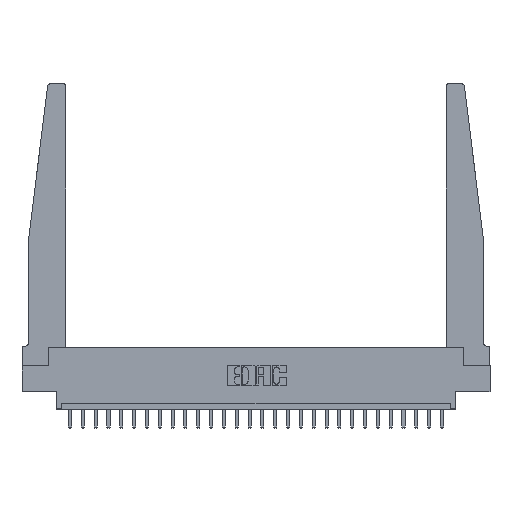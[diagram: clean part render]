
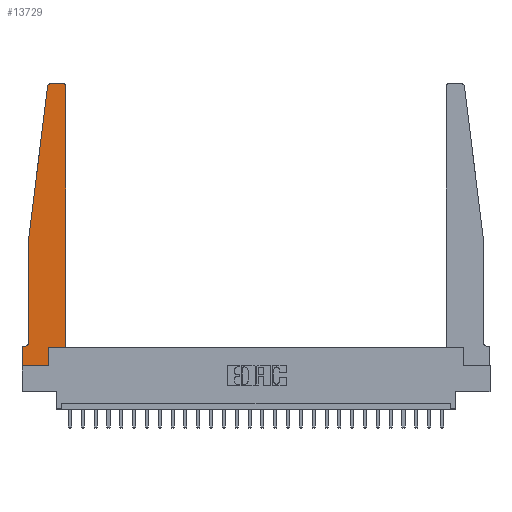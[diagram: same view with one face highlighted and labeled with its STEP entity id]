
A CAD part, top view. The second image highlights one B-rep face of the part: STEP entity #13729.
In plain terms, the highlighted planar face has unit normal (0, 0, 1).
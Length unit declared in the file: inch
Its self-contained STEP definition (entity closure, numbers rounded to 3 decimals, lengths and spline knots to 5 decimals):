
#373 = ORIENTED_EDGE ( 'NONE', *, *, #19788, .T. ) ;
#397 = CARTESIAN_POINT ( 'NONE',  ( 0.27653, 2.72, 0.37 ) ) ;
#616 = AXIS2_PLACEMENT_3D ( 'NONE', #15666, #13822, #25387 ) ;
#745 = LINE ( 'NONE', #6727, #14273 ) ;
#876 = VERTEX_POINT ( 'NONE', #17961 ) ;
#1001 = DIRECTION ( 'NONE',  ( 0., -1., 0. ) ) ;
#1969 = EDGE_CURVE ( 'NONE', #15614, #10396, #3071, .T. ) ;
#2006 = CARTESIAN_POINT ( 'NONE',  ( 0.065, 0.2375, 0.37 ) ) ;
#2117 = LINE ( 'NONE', #25653, #13832 ) ;
#2193 = VERTEX_POINT ( 'NONE', #17862 ) ;
#2628 = AXIS2_PLACEMENT_3D ( 'NONE', #17552, #11711, #25481 ) ;
#2677 = EDGE_CURVE ( 'NONE', #2193, #18642, #17796, .T. ) ;
#3039 = VECTOR ( 'NONE', #8495, 39.37008 ) ;
#3071 = LINE ( 'NONE', #18653, #11666 ) ;
#3136 = VECTOR ( 'NONE', #12286, 39.37008 ) ;
#3197 = ORIENTED_EDGE ( 'NONE', *, *, #13480, .T. ) ;
#3854 = VERTEX_POINT ( 'NONE', #13686 ) ;
#3909 = CARTESIAN_POINT ( 'NONE',  ( 0.425, 0.18, 0.37 ) ) ;
#4334 = ORIENTED_EDGE ( 'NONE', *, *, #24611, .T. ) ;
#4582 = FACE_OUTER_BOUND ( 'NONE', #11427, .T. ) ;
#4681 = ORIENTED_EDGE ( 'NONE', *, *, #14001, .T. ) ;
#4750 = CIRCLE ( 'NONE', #616, 0.03 ) ;
#5121 = ORIENTED_EDGE ( 'NONE', *, *, #21421, .T. ) ;
#6515 = DIRECTION ( 'NONE',  ( 0., 0., 1. ) ) ;
#6606 = CARTESIAN_POINT ( 'NONE',  ( 0.2605, 0.18, 0.37 ) ) ;
#6727 = CARTESIAN_POINT ( 'NONE',  ( 0.425, 0.18, 0.37 ) ) ;
#6967 = CARTESIAN_POINT ( 'NONE',  ( 0.2605, 0.18, 0.37 ) ) ;
#7396 = LINE ( 'NONE', #15320, #24579 ) ;
#7445 = CARTESIAN_POINT ( 'NONE',  ( 0.395, 2.75, 0.37 ) ) ;
#7620 = CIRCLE ( 'NONE', #2628, 0.05 ) ;
#8340 = CARTESIAN_POINT ( 'NONE',  ( 0.015, 0.1875, 0.37 ) ) ;
#8495 = DIRECTION ( 'NONE',  ( 1., 0., 0. ) ) ;
#8884 = ORIENTED_EDGE ( 'NONE', *, *, #10788, .T. ) ;
#9213 = DIRECTION ( 'NONE',  ( 0., 0., 1. ) ) ;
#10092 = CARTESIAN_POINT ( 'NONE',  ( 0.425, 2.72, 0.37 ) ) ;
#10161 = EDGE_CURVE ( 'NONE', #19123, #22030, #7620, .T. ) ;
#10373 = DIRECTION ( 'NONE',  ( 0., 1., 0. ) ) ;
#10396 = VERTEX_POINT ( 'NONE', #3909 ) ;
#10788 = EDGE_CURVE ( 'NONE', #10396, #21127, #745, .T. ) ;
#10823 = CARTESIAN_POINT ( 'NONE',  ( 0.2605, 0., 0.37 ) ) ;
#10944 = CARTESIAN_POINT ( 'NONE',  ( 0., 0., 0.37 ) ) ;
#11157 = AXIS2_PLACEMENT_3D ( 'NONE', #397, #6515, #16243 ) ;
#11427 = EDGE_LOOP ( 'NONE', ( #23142, #13453, #373, #4334, #13559, #3197, #15904, #20537, #4681, #17991, #8884, #5121 ) ) ;
#11666 = VECTOR ( 'NONE', #16470, 39.37008 ) ;
#11711 = DIRECTION ( 'NONE',  ( 0., 0., -1. ) ) ;
#12286 = DIRECTION ( 'NONE',  ( -1., 0., 0. ) ) ;
#13453 = ORIENTED_EDGE ( 'NONE', *, *, #2677, .T. ) ;
#13480 = EDGE_CURVE ( 'NONE', #22030, #14631, #14989, .T. ) ;
#13559 = ORIENTED_EDGE ( 'NONE', *, *, #10161, .T. ) ;
#13686 = CARTESIAN_POINT ( 'NONE',  ( 0., 0., 0.37 ) ) ;
#13729 = ADVANCED_FACE ( 'NONE', ( #4582 ), #22475, .T. ) ;
#13822 = DIRECTION ( 'NONE',  ( 0., 0., 1. ) ) ;
#13832 = VECTOR ( 'NONE', #14084, 39.37008 ) ;
#14001 = EDGE_CURVE ( 'NONE', #22856, #15614, #16473, .T. ) ;
#14084 = DIRECTION ( 'NONE',  ( 0., -1., 0. ) ) ;
#14273 = VECTOR ( 'NONE', #22545, 39.37008 ) ;
#14631 = VERTEX_POINT ( 'NONE', #19500 ) ;
#14854 = LINE ( 'NONE', #10944, #3039 ) ;
#14989 = LINE ( 'NONE', #20952, #18091 ) ;
#15122 = DIRECTION ( 'NONE',  ( -1., 0., 0. ) ) ;
#15217 = VECTOR ( 'NONE', #10373, 39.37008 ) ;
#15320 = CARTESIAN_POINT ( 'NONE',  ( 0.065, 1.25, 0.37 ) ) ;
#15614 = VERTEX_POINT ( 'NONE', #6967 ) ;
#15666 = CARTESIAN_POINT ( 'NONE',  ( 0.395, 2.72, 0.37 ) ) ;
#15904 = ORIENTED_EDGE ( 'NONE', *, *, #20406, .T. ) ;
#16202 = VERTEX_POINT ( 'NONE', #7445 ) ;
#16243 = DIRECTION ( 'NONE',  ( 1., 0., 0. ) ) ;
#16470 = DIRECTION ( 'NONE',  ( 1., 0., 0. ) ) ;
#16473 = LINE ( 'NONE', #6606, #15217 ) ;
#17244 = VECTOR ( 'NONE', #1001, 39.37008 ) ;
#17552 = CARTESIAN_POINT ( 'NONE',  ( 0.015, 0.2375, 0.37 ) ) ;
#17796 = CIRCLE ( 'NONE', #11157, 0.03 ) ;
#17862 = CARTESIAN_POINT ( 'NONE',  ( 0.27653, 2.75, 0.37 ) ) ;
#17961 = CARTESIAN_POINT ( 'NONE',  ( 0.065, 1.25, 0.37 ) ) ;
#17991 = ORIENTED_EDGE ( 'NONE', *, *, #1969, .T. ) ;
#18091 = VECTOR ( 'NONE', #15122, 39.37008 ) ;
#18593 = DIRECTION ( 'NONE',  ( 1., 0., 0. ) ) ;
#18642 = VERTEX_POINT ( 'NONE', #24704 ) ;
#18653 = CARTESIAN_POINT ( 'NONE',  ( 0.425, 0.18, 0.37 ) ) ;
#18786 = LINE ( 'NONE', #24904, #17244 ) ;
#19123 = VERTEX_POINT ( 'NONE', #2006 ) ;
#19500 = CARTESIAN_POINT ( 'NONE',  ( 0., 0.1875, 0.37 ) ) ;
#19788 = EDGE_CURVE ( 'NONE', #18642, #876, #7396, .T. ) ;
#20406 = EDGE_CURVE ( 'NONE', #14631, #3854, #2117, .T. ) ;
#20537 = ORIENTED_EDGE ( 'NONE', *, *, #20574, .T. ) ;
#20574 = EDGE_CURVE ( 'NONE', #3854, #22856, #14854, .T. ) ;
#20952 = CARTESIAN_POINT ( 'NONE',  ( 0.065, 0.1875, 0.37 ) ) ;
#21127 = VERTEX_POINT ( 'NONE', #10092 ) ;
#21421 = EDGE_CURVE ( 'NONE', #21127, #16202, #4750, .T. ) ;
#21989 = LINE ( 'NONE', #22118, #3136 ) ;
#22030 = VERTEX_POINT ( 'NONE', #8340 ) ;
#22118 = CARTESIAN_POINT ( 'NONE',  ( 0.25, 2.75, 0.37 ) ) ;
#22240 = CARTESIAN_POINT ( 'NONE',  ( 0., 0.1875, 0.37 ) ) ;
#22475 = PLANE ( 'NONE',  #25168 ) ;
#22545 = DIRECTION ( 'NONE',  ( 0., 1., 0. ) ) ;
#22721 = EDGE_CURVE ( 'NONE', #16202, #2193, #21989, .T. ) ;
#22856 = VERTEX_POINT ( 'NONE', #10823 ) ;
#23142 = ORIENTED_EDGE ( 'NONE', *, *, #22721, .T. ) ;
#23211 = DIRECTION ( 'NONE',  ( -0.122, -0.992, 0. ) ) ;
#24579 = VECTOR ( 'NONE', #23211, 39.37008 ) ;
#24611 = EDGE_CURVE ( 'NONE', #876, #19123, #18786, .T. ) ;
#24704 = CARTESIAN_POINT ( 'NONE',  ( 0.24675, 2.72367, 0.37 ) ) ;
#24904 = CARTESIAN_POINT ( 'NONE',  ( 0.065, 1.25, 0.37 ) ) ;
#25168 = AXIS2_PLACEMENT_3D ( 'NONE', #22240, #9213, #18593 ) ;
#25387 = DIRECTION ( 'NONE',  ( 1., 0., 0. ) ) ;
#25481 = DIRECTION ( 'NONE',  ( -1., 0., 0. ) ) ;
#25653 = CARTESIAN_POINT ( 'NONE',  ( 0., 0., 0.37 ) ) ;
